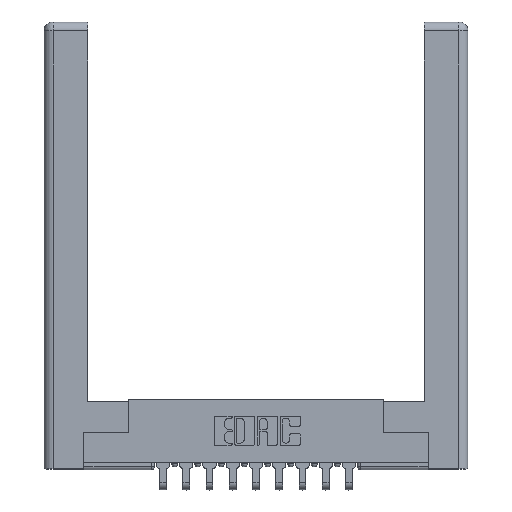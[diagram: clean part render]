
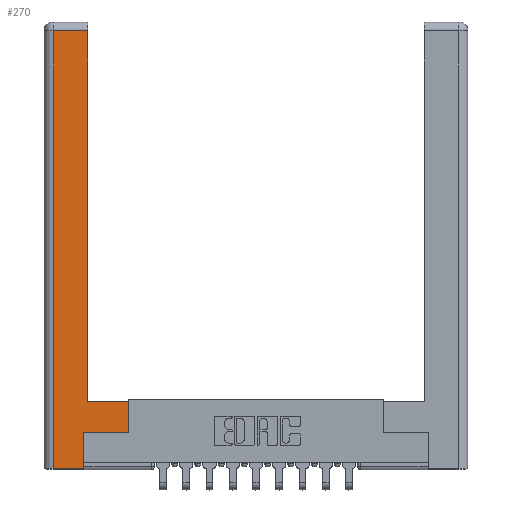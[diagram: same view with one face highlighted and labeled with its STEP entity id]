
A CAD part, top view. The second image highlights one B-rep face of the part: STEP entity #270.
In plain terms, the highlighted planar face has unit normal (0, 0, 1).
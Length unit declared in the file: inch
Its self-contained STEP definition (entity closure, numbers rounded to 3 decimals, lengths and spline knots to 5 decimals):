
#17 = FACE_OUTER_BOUND ( 'NONE', #9488, .T. ) ;
#223 = DIRECTION ( 'NONE',  ( 0., 0., -1. ) ) ;
#270 = ADVANCED_FACE ( 'NONE', ( #17 ), #11590, .F. ) ;
#332 = ORIENTED_EDGE ( 'NONE', *, *, #13518, .T. ) ;
#598 = CARTESIAN_POINT ( 'NONE',  ( 0.565, 0.245, 0. ) ) ;
#850 = ORIENTED_EDGE ( 'NONE', *, *, #2798, .T. ) ;
#1044 = VECTOR ( 'NONE', #6674, 39.37008 ) ;
#1045 = ORIENTED_EDGE ( 'NONE', *, *, #13411, .T. ) ;
#1156 = DIRECTION ( 'NONE',  ( 0., 1., 0. ) ) ;
#1548 = DIRECTION ( 'NONE',  ( 0., 1., 0. ) ) ;
#1665 = LINE ( 'NONE', #7051, #5504 ) ;
#1737 = CARTESIAN_POINT ( 'NONE',  ( 0.0615, 0., 0. ) ) ;
#1886 = CARTESIAN_POINT ( 'NONE',  ( 0.295, 0.45, 0. ) ) ;
#1893 = EDGE_CURVE ( 'NONE', #4571, #9033, #9130, .T. ) ;
#1953 = VERTEX_POINT ( 'NONE', #4361 ) ;
#1960 = VERTEX_POINT ( 'NONE', #14459 ) ;
#2309 = VERTEX_POINT ( 'NONE', #598 ) ;
#2631 = VERTEX_POINT ( 'NONE', #7884 ) ;
#2788 = VECTOR ( 'NONE', #2871, 39.37008 ) ;
#2798 = EDGE_CURVE ( 'NONE', #1960, #2309, #4460, .T. ) ;
#2871 = DIRECTION ( 'NONE',  ( -1., 0., 0. ) ) ;
#3115 = DIRECTION ( 'NONE',  ( -1., 0., 0. ) ) ;
#3392 = ORIENTED_EDGE ( 'NONE', *, *, #6137, .T. ) ;
#4361 = CARTESIAN_POINT ( 'NONE',  ( 0.295, 0.45, 0. ) ) ;
#4460 = LINE ( 'NONE', #5817, #7620 ) ;
#4571 = VERTEX_POINT ( 'NONE', #6795 ) ;
#4815 = VECTOR ( 'NONE', #1156, 39.37008 ) ;
#5402 = LINE ( 'NONE', #10550, #6833 ) ;
#5504 = VECTOR ( 'NONE', #1548, 39.37008 ) ;
#5560 = AXIS2_PLACEMENT_3D ( 'NONE', #9392, #223, #9206 ) ;
#5708 = CARTESIAN_POINT ( 'NONE',  ( 0.565, 0.45, 0. ) ) ;
#5773 = LINE ( 'NONE', #12057, #2788 ) ;
#5817 = CARTESIAN_POINT ( 'NONE',  ( 0.565, 0.245, 0. ) ) ;
#6137 = EDGE_CURVE ( 'NONE', #8430, #4571, #5773, .T. ) ;
#6572 = CARTESIAN_POINT ( 'NONE',  ( 0.0615, 0., 0. ) ) ;
#6674 = DIRECTION ( 'NONE',  ( 0., -1., 0. ) ) ;
#6795 = CARTESIAN_POINT ( 'NONE',  ( 0.0615, 2.94, 0. ) ) ;
#6833 = VECTOR ( 'NONE', #12026, 39.37008 ) ;
#7051 = CARTESIAN_POINT ( 'NONE',  ( 0.265, 0.245, 0. ) ) ;
#7136 = ORIENTED_EDGE ( 'NONE', *, *, #12117, .T. ) ;
#7620 = VECTOR ( 'NONE', #8235, 39.37008 ) ;
#7851 = VECTOR ( 'NONE', #3115, 39.37008 ) ;
#7884 = CARTESIAN_POINT ( 'NONE',  ( 0.265, 0., 0. ) ) ;
#7917 = ORIENTED_EDGE ( 'NONE', *, *, #10850, .T. ) ;
#8235 = DIRECTION ( 'NONE',  ( 1., 0., 0. ) ) ;
#8249 = CARTESIAN_POINT ( 'NONE',  ( 0.295, 2.94, 0. ) ) ;
#8430 = VERTEX_POINT ( 'NONE', #8249 ) ;
#8850 = VERTEX_POINT ( 'NONE', #11256 ) ;
#8903 = LINE ( 'NONE', #1886, #7851 ) ;
#9033 = VERTEX_POINT ( 'NONE', #1737 ) ;
#9130 = LINE ( 'NONE', #6572, #1044 ) ;
#9206 = DIRECTION ( 'NONE',  ( -1., 0., 0. ) ) ;
#9392 = CARTESIAN_POINT ( 'NONE',  ( 0., 0., 0. ) ) ;
#9488 = EDGE_LOOP ( 'NONE', ( #7917, #3392, #13491, #9585, #332, #850, #1045, #7136 ) ) ;
#9565 = LINE ( 'NONE', #5708, #4815 ) ;
#9585 = ORIENTED_EDGE ( 'NONE', *, *, #11338, .T. ) ;
#10550 = CARTESIAN_POINT ( 'NONE',  ( 0.265, 0., 0. ) ) ;
#10843 = DIRECTION ( 'NONE',  ( 0., 1., 0. ) ) ;
#10850 = EDGE_CURVE ( 'NONE', #1953, #8430, #13681, .T. ) ;
#11256 = CARTESIAN_POINT ( 'NONE',  ( 0.565, 0.45, 0. ) ) ;
#11338 = EDGE_CURVE ( 'NONE', #9033, #2631, #5402, .T. ) ;
#11590 = PLANE ( 'NONE',  #5560 ) ;
#11936 = VECTOR ( 'NONE', #10843, 39.37008 ) ;
#12026 = DIRECTION ( 'NONE',  ( 1., 0., 0. ) ) ;
#12057 = CARTESIAN_POINT ( 'NONE',  ( 0.0615, 2.94, 0. ) ) ;
#12117 = EDGE_CURVE ( 'NONE', #8850, #1953, #8903, .T. ) ;
#13206 = CARTESIAN_POINT ( 'NONE',  ( 0.295, 3., 0. ) ) ;
#13411 = EDGE_CURVE ( 'NONE', #2309, #8850, #9565, .T. ) ;
#13491 = ORIENTED_EDGE ( 'NONE', *, *, #1893, .T. ) ;
#13518 = EDGE_CURVE ( 'NONE', #2631, #1960, #1665, .T. ) ;
#13681 = LINE ( 'NONE', #13206, #11936 ) ;
#14459 = CARTESIAN_POINT ( 'NONE',  ( 0.265, 0.245, 0. ) ) ;
